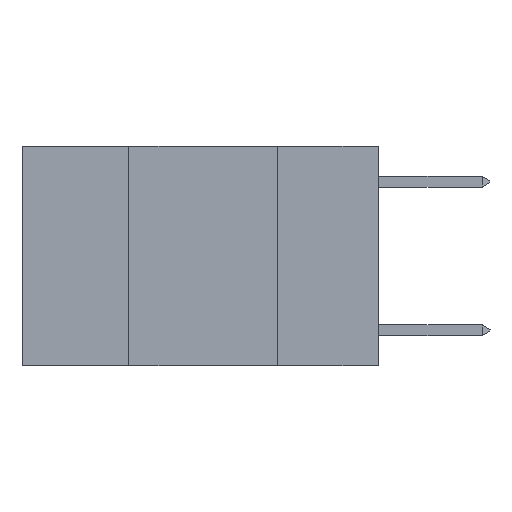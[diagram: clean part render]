
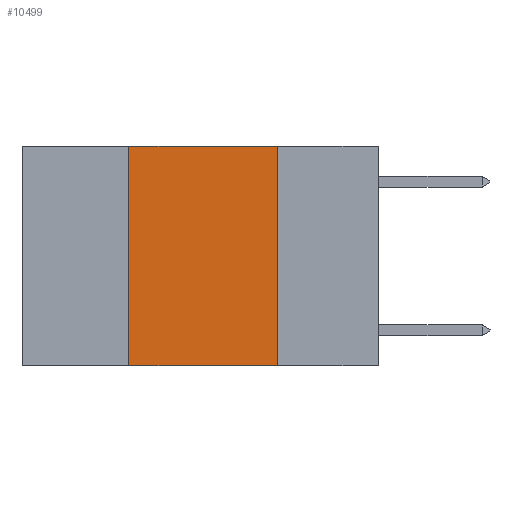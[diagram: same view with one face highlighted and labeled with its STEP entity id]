
A CAD part, left-side view. The second image highlights one B-rep face of the part: STEP entity #10499.
In plain terms, the highlighted planar face has unit normal (-1, 0, 0).
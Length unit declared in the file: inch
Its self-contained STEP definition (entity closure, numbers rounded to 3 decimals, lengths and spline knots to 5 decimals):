
#194 = ORIENTED_EDGE ( 'NONE', *, *, #10350, .F. ) ;
#474 = CARTESIAN_POINT ( 'NONE',  ( 0., 0.6, 0. ) ) ;
#1594 = DIRECTION ( 'NONE',  ( 0., -1., 0. ) ) ;
#3176 = ORIENTED_EDGE ( 'NONE', *, *, #8448, .F. ) ;
#3219 = CARTESIAN_POINT ( 'NONE',  ( 0., 0.42, -0.37 ) ) ;
#3655 = DIRECTION ( 'NONE',  ( 0., 0., 1. ) ) ;
#3781 = VERTEX_POINT ( 'NONE', #4252 ) ;
#3878 = EDGE_CURVE ( 'NONE', #6179, #8608, #9186, .T. ) ;
#4252 = CARTESIAN_POINT ( 'NONE',  ( 0., 0.17, 0. ) ) ;
#4400 = DIRECTION ( 'NONE',  ( 0., -1., 0. ) ) ;
#6099 = VECTOR ( 'NONE', #8646, 39.37008 ) ;
#6179 = VERTEX_POINT ( 'NONE', #3219 ) ;
#6428 = EDGE_CURVE ( 'NONE', #6179, #12226, #10662, .T. ) ;
#6568 = CARTESIAN_POINT ( 'NONE',  ( 0., 0.42, 0. ) ) ;
#6708 = DIRECTION ( 'NONE',  ( 0., 0., -1. ) ) ;
#6793 = LINE ( 'NONE', #9697, #6099 ) ;
#7541 = LINE ( 'NONE', #474, #13610 ) ;
#8448 = EDGE_CURVE ( 'NONE', #12226, #3781, #7541, .T. ) ;
#8608 = VERTEX_POINT ( 'NONE', #11781 ) ;
#8646 = DIRECTION ( 'NONE',  ( 0., 0., -1. ) ) ;
#8761 = ORIENTED_EDGE ( 'NONE', *, *, #3878, .T. ) ;
#8825 = CARTESIAN_POINT ( 'NONE',  ( 0., 0.6, -0.37 ) ) ;
#8853 = VECTOR ( 'NONE', #4400, 39.37008 ) ;
#8874 = PLANE ( 'NONE',  #9572 ) ;
#9186 = LINE ( 'NONE', #8825, #8853 ) ;
#9572 = AXIS2_PLACEMENT_3D ( 'NONE', #11029, #13191, #6708 ) ;
#9697 = CARTESIAN_POINT ( 'NONE',  ( 0., 0.17, 0. ) ) ;
#9872 = FACE_OUTER_BOUND ( 'NONE', #14212, .T. ) ;
#10350 = EDGE_CURVE ( 'NONE', #3781, #8608, #6793, .T. ) ;
#10499 = ADVANCED_FACE ( 'NONE', ( #9872 ), #8874, .F. ) ;
#10662 = LINE ( 'NONE', #13505, #13502 ) ;
#11029 = CARTESIAN_POINT ( 'NONE',  ( 0., 0.6, 0. ) ) ;
#11781 = CARTESIAN_POINT ( 'NONE',  ( 0., 0.17, -0.37 ) ) ;
#12226 = VERTEX_POINT ( 'NONE', #6568 ) ;
#13191 = DIRECTION ( 'NONE',  ( 1., 0., 0. ) ) ;
#13502 = VECTOR ( 'NONE', #3655, 39.37008 ) ;
#13505 = CARTESIAN_POINT ( 'NONE',  ( 0., 0.42, 0. ) ) ;
#13610 = VECTOR ( 'NONE', #1594, 39.37008 ) ;
#14107 = ORIENTED_EDGE ( 'NONE', *, *, #6428, .F. ) ;
#14212 = EDGE_LOOP ( 'NONE', ( #194, #3176, #14107, #8761 ) ) ;
